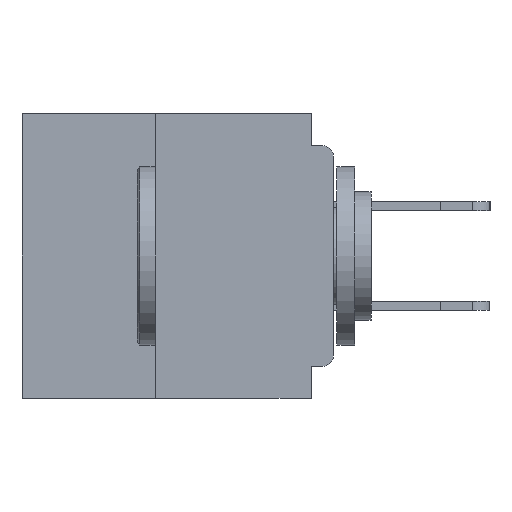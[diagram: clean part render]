
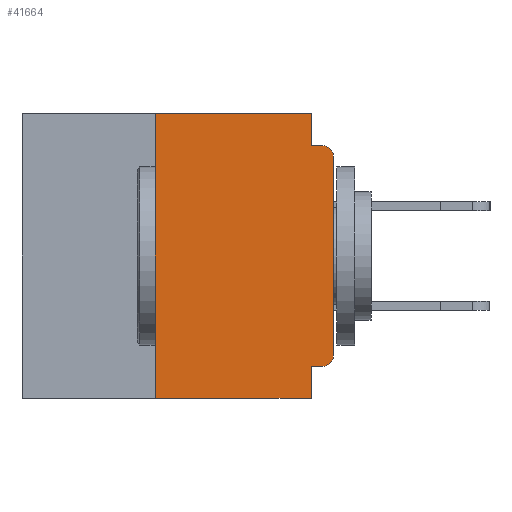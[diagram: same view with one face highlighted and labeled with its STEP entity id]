
A CAD part, left-side view. The second image highlights one B-rep face of the part: STEP entity #41664.
In plain terms, the highlighted planar face has unit normal (-1, 0, 0).
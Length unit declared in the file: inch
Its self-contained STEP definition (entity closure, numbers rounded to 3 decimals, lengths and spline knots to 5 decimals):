
#11 = CARTESIAN_POINT ( 'NONE',  ( 0., 0., -0.045 ) ) ;
#991 = PLANE ( 'NONE',  #10425 ) ;
#999 = VECTOR ( 'NONE', #28246, 39.37008 ) ;
#2147 = AXIS2_PLACEMENT_3D ( 'NONE', #8941, #35176, #12739 ) ;
#3650 = LINE ( 'NONE', #28330, #32427 ) ;
#4164 = EDGE_CURVE ( 'NONE', #47994, #5789, #27041, .T. ) ;
#4419 = CARTESIAN_POINT ( 'NONE',  ( 0., 0., -0.34 ) ) ;
#4616 = VERTEX_POINT ( 'NONE', #4419 ) ;
#4859 = CARTESIAN_POINT ( 'NONE',  ( 0., 0.437, 0. ) ) ;
#5789 = VERTEX_POINT ( 'NONE', #31463 ) ;
#6488 = CARTESIAN_POINT ( 'NONE',  ( 0., 0.25, -0.4 ) ) ;
#6594 = LINE ( 'NONE', #39346, #24223 ) ;
#8594 = DIRECTION ( 'NONE',  ( 1., 0., 0. ) ) ;
#8941 = CARTESIAN_POINT ( 'NONE',  ( 0., 0.015, -0.34 ) ) ;
#9043 = LINE ( 'NONE', #6488, #47739 ) ;
#9491 = DIRECTION ( 'NONE',  ( 0., 1., 0. ) ) ;
#9603 = LINE ( 'NONE', #39743, #48310 ) ;
#10425 = AXIS2_PLACEMENT_3D ( 'NONE', #4859, #8594, #34839 ) ;
#11156 = ORIENTED_EDGE ( 'NONE', *, *, #12363, .T. ) ;
#11490 = CARTESIAN_POINT ( 'NONE',  ( 0., 0.25, 0. ) ) ;
#11738 = ORIENTED_EDGE ( 'NONE', *, *, #38862, .F. ) ;
#11966 = DIRECTION ( 'NONE',  ( 0., 0., -1. ) ) ;
#11981 = VECTOR ( 'NONE', #11966, 39.37008 ) ;
#12363 = EDGE_CURVE ( 'NONE', #37300, #18291, #3650, .T. ) ;
#12425 = CARTESIAN_POINT ( 'NONE',  ( 0., 0.015, -0.355 ) ) ;
#12739 = DIRECTION ( 'NONE',  ( 0., 0., -1. ) ) ;
#13062 = DIRECTION ( 'NONE',  ( 0., 0., 1. ) ) ;
#14422 = CARTESIAN_POINT ( 'NONE',  ( 0., 0., -0.06 ) ) ;
#16981 = FACE_OUTER_BOUND ( 'NONE', #25985, .T. ) ;
#17994 = DIRECTION ( 'NONE',  ( 0., 0., -1. ) ) ;
#18029 = DIRECTION ( 'NONE',  ( -1., 0., 0. ) ) ;
#18035 = CARTESIAN_POINT ( 'NONE',  ( 0., 0.015, -0.06 ) ) ;
#18291 = VERTEX_POINT ( 'NONE', #45182 ) ;
#18368 = VECTOR ( 'NONE', #22572, 39.37008 ) ;
#20129 = EDGE_CURVE ( 'NONE', #37300, #33475, #9043, .T. ) ;
#20401 = EDGE_CURVE ( 'NONE', #34733, #4616, #45955, .T. ) ;
#21069 = DIRECTION ( 'NONE',  ( 0., -1., 0. ) ) ;
#21729 = CARTESIAN_POINT ( 'NONE',  ( 0., 0.031, -0.355 ) ) ;
#22221 = ORIENTED_EDGE ( 'NONE', *, *, #20401, .T. ) ;
#22572 = DIRECTION ( 'NONE',  ( 0., -1., 0. ) ) ;
#23190 = ORIENTED_EDGE ( 'NONE', *, *, #39393, .F. ) ;
#23503 = VERTEX_POINT ( 'NONE', #21729 ) ;
#24062 = CARTESIAN_POINT ( 'NONE',  ( 0., 0.031, -0.045 ) ) ;
#24223 = VECTOR ( 'NONE', #9491, 39.37008 ) ;
#24478 = ORIENTED_EDGE ( 'NONE', *, *, #44885, .T. ) ;
#25322 = ORIENTED_EDGE ( 'NONE', *, *, #4164, .T. ) ;
#25985 = EDGE_LOOP ( 'NONE', ( #24478, #25322, #23190, #26466, #43728, #38037, #11156, #11738, #45895, #22221 ) ) ;
#26466 = ORIENTED_EDGE ( 'NONE', *, *, #31335, .F. ) ;
#27041 = CIRCLE ( 'NONE', #30278, 0.015 ) ;
#27937 = VERTEX_POINT ( 'NONE', #35113 ) ;
#28069 = EDGE_CURVE ( 'NONE', #33475, #27937, #9603, .T. ) ;
#28246 = DIRECTION ( 'NONE',  ( 0., 0., -1. ) ) ;
#28318 = CARTESIAN_POINT ( 'NONE',  ( 0., 0.25, -0.4 ) ) ;
#28330 = CARTESIAN_POINT ( 'NONE',  ( 0., 0.437, -0.4 ) ) ;
#30278 = AXIS2_PLACEMENT_3D ( 'NONE', #18035, #18029, #17994 ) ;
#30587 = LINE ( 'NONE', #31738, #40496 ) ;
#31335 = EDGE_CURVE ( 'NONE', #27937, #34772, #32156, .T. ) ;
#31463 = CARTESIAN_POINT ( 'NONE',  ( 0., 0.015, -0.045 ) ) ;
#31738 = CARTESIAN_POINT ( 'NONE',  ( 0., 0., 0. ) ) ;
#31913 = LINE ( 'NONE', #34424, #11981 ) ;
#32156 = LINE ( 'NONE', #35611, #999 ) ;
#32427 = VECTOR ( 'NONE', #39637, 39.37008 ) ;
#32734 = DIRECTION ( 'NONE',  ( 0., 0., 1. ) ) ;
#33475 = VERTEX_POINT ( 'NONE', #11490 ) ;
#33781 = EDGE_CURVE ( 'NONE', #34733, #23503, #6594, .T. ) ;
#34424 = CARTESIAN_POINT ( 'NONE',  ( 0., 0.031, -0.4 ) ) ;
#34733 = VERTEX_POINT ( 'NONE', #12425 ) ;
#34772 = VERTEX_POINT ( 'NONE', #24062 ) ;
#34839 = DIRECTION ( 'NONE',  ( 0., 0., -1. ) ) ;
#35113 = CARTESIAN_POINT ( 'NONE',  ( 0., 0.031, 0. ) ) ;
#35176 = DIRECTION ( 'NONE',  ( -1., 0., 0. ) ) ;
#35611 = CARTESIAN_POINT ( 'NONE',  ( 0., 0.031, 0. ) ) ;
#37300 = VERTEX_POINT ( 'NONE', #28318 ) ;
#38037 = ORIENTED_EDGE ( 'NONE', *, *, #20129, .F. ) ;
#38317 = LINE ( 'NONE', #11, #18368 ) ;
#38862 = EDGE_CURVE ( 'NONE', #23503, #18291, #31913, .T. ) ;
#39346 = CARTESIAN_POINT ( 'NONE',  ( 0., 0., -0.355 ) ) ;
#39393 = EDGE_CURVE ( 'NONE', #34772, #5789, #38317, .T. ) ;
#39637 = DIRECTION ( 'NONE',  ( 0., -1., 0. ) ) ;
#39743 = CARTESIAN_POINT ( 'NONE',  ( 0., 0.437, 0. ) ) ;
#40496 = VECTOR ( 'NONE', #13062, 39.37008 ) ;
#41664 = ADVANCED_FACE ( 'NONE', ( #16981 ), #991, .F. ) ;
#43728 = ORIENTED_EDGE ( 'NONE', *, *, #28069, .F. ) ;
#44885 = EDGE_CURVE ( 'NONE', #4616, #47994, #30587, .T. ) ;
#45182 = CARTESIAN_POINT ( 'NONE',  ( 0., 0.031, -0.4 ) ) ;
#45895 = ORIENTED_EDGE ( 'NONE', *, *, #33781, .F. ) ;
#45955 = CIRCLE ( 'NONE', #2147, 0.015 ) ;
#47739 = VECTOR ( 'NONE', #32734, 39.37008 ) ;
#47994 = VERTEX_POINT ( 'NONE', #14422 ) ;
#48310 = VECTOR ( 'NONE', #21069, 39.37008 ) ;
